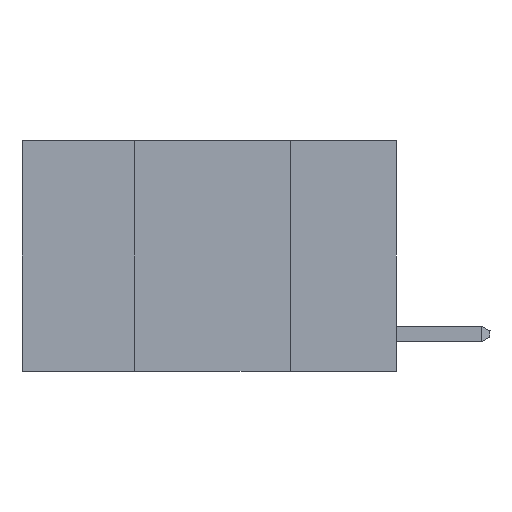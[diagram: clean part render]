
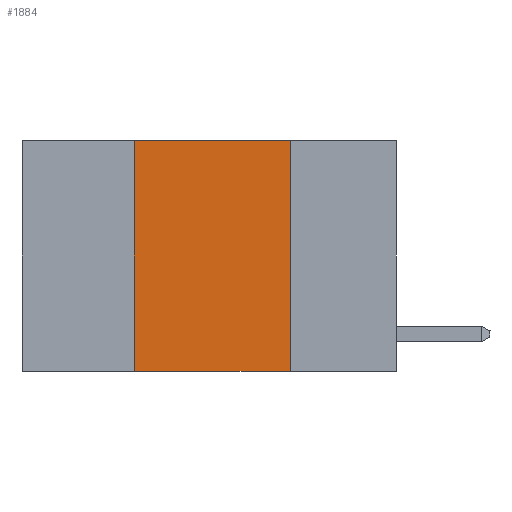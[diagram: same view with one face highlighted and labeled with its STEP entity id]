
A CAD part, left-side view. The second image highlights one B-rep face of the part: STEP entity #1884.
In plain terms, the highlighted planar face has unit normal (-1, 0, 0).
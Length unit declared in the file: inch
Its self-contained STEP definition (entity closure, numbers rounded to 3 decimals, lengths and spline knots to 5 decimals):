
#256 = FACE_OUTER_BOUND ( 'NONE', #1828, .T. ) ;
#729 = LINE ( 'NONE', #4529, #8555 ) ;
#887 = LINE ( 'NONE', #12785, #15133 ) ;
#920 = EDGE_CURVE ( 'NONE', #4064, #8558, #15410, .T. ) ;
#932 = DIRECTION ( 'NONE',  ( 0., 0., 1. ) ) ;
#1187 = CARTESIAN_POINT ( 'NONE',  ( 0., 0.42, 0. ) ) ;
#1622 = CARTESIAN_POINT ( 'NONE',  ( 0., 0.42, -0.37 ) ) ;
#1828 = EDGE_LOOP ( 'NONE', ( #5557, #10583, #12309, #16969 ) ) ;
#1838 = AXIS2_PLACEMENT_3D ( 'NONE', #6899, #9495, #16037 ) ;
#1884 = ADVANCED_FACE ( 'NONE', ( #256 ), #14472, .F. ) ;
#3394 = EDGE_CURVE ( 'NONE', #8558, #10418, #887, .T. ) ;
#3986 = VERTEX_POINT ( 'NONE', #15583 ) ;
#4064 = VERTEX_POINT ( 'NONE', #1622 ) ;
#4529 = CARTESIAN_POINT ( 'NONE',  ( 0., 0.6, -0.37 ) ) ;
#4691 = DIRECTION ( 'NONE',  ( 0., -1., 0. ) ) ;
#5557 = ORIENTED_EDGE ( 'NONE', *, *, #10749, .F. ) ;
#6899 = CARTESIAN_POINT ( 'NONE',  ( 0., 0.6, 0. ) ) ;
#7222 = VECTOR ( 'NONE', #932, 39.37008 ) ;
#7309 = CARTESIAN_POINT ( 'NONE',  ( 0., 0.17, 0. ) ) ;
#8456 = CARTESIAN_POINT ( 'NONE',  ( 0., 0.42, 0. ) ) ;
#8555 = VECTOR ( 'NONE', #9866, 39.37008 ) ;
#8558 = VERTEX_POINT ( 'NONE', #8456 ) ;
#9495 = DIRECTION ( 'NONE',  ( 1., 0., 0. ) ) ;
#9632 = CARTESIAN_POINT ( 'NONE',  ( 0., 0.17, 0. ) ) ;
#9719 = LINE ( 'NONE', #9632, #13649 ) ;
#9866 = DIRECTION ( 'NONE',  ( 0., -1., 0. ) ) ;
#10418 = VERTEX_POINT ( 'NONE', #7309 ) ;
#10583 = ORIENTED_EDGE ( 'NONE', *, *, #3394, .F. ) ;
#10749 = EDGE_CURVE ( 'NONE', #10418, #3986, #9719, .T. ) ;
#12309 = ORIENTED_EDGE ( 'NONE', *, *, #920, .F. ) ;
#12785 = CARTESIAN_POINT ( 'NONE',  ( 0., 0.6, 0. ) ) ;
#13495 = DIRECTION ( 'NONE',  ( 0., 0., -1. ) ) ;
#13649 = VECTOR ( 'NONE', #13495, 39.37008 ) ;
#14472 = PLANE ( 'NONE',  #1838 ) ;
#14686 = EDGE_CURVE ( 'NONE', #4064, #3986, #729, .T. ) ;
#15133 = VECTOR ( 'NONE', #4691, 39.37008 ) ;
#15410 = LINE ( 'NONE', #1187, #7222 ) ;
#15583 = CARTESIAN_POINT ( 'NONE',  ( 0., 0.17, -0.37 ) ) ;
#16037 = DIRECTION ( 'NONE',  ( 0., 0., -1. ) ) ;
#16969 = ORIENTED_EDGE ( 'NONE', *, *, #14686, .T. ) ;
